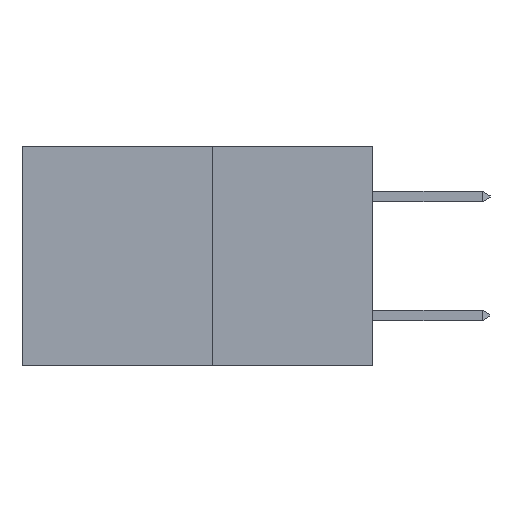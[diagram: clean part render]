
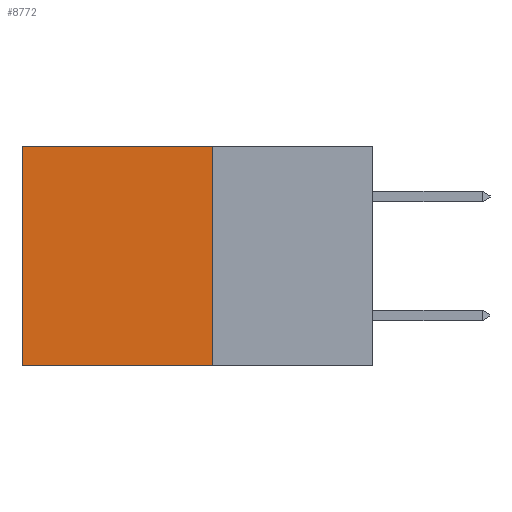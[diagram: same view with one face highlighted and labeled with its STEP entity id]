
A CAD part, left-side view. The second image highlights one B-rep face of the part: STEP entity #8772.
In plain terms, the highlighted planar face has unit normal (-1, 0, 0).
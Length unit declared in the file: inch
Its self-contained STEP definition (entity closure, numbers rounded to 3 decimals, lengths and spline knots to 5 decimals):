
#149 = VERTEX_POINT ( 'NONE', #5494 ) ;
#459 = ORIENTED_EDGE ( 'NONE', *, *, #4721, .F. ) ;
#1089 = VERTEX_POINT ( 'NONE', #6382 ) ;
#1174 = CARTESIAN_POINT ( 'NONE',  ( 0.277, 0.27, 0. ) ) ;
#1206 = CARTESIAN_POINT ( 'NONE',  ( 0.277, 0.27, -0.37 ) ) ;
#1286 = LINE ( 'NONE', #1206, #12986 ) ;
#1322 = EDGE_CURVE ( 'NONE', #11933, #1089, #7923, .T. ) ;
#1432 = CARTESIAN_POINT ( 'NONE',  ( 0.277, 0.59, 0. ) ) ;
#1662 = VECTOR ( 'NONE', #5779, 39.37008 ) ;
#2439 = CARTESIAN_POINT ( 'NONE',  ( 0.277, 0.27, -0.37 ) ) ;
#2505 = PLANE ( 'NONE',  #3910 ) ;
#2763 = EDGE_LOOP ( 'NONE', ( #3074, #7607, #459, #6108 ) ) ;
#2765 = VECTOR ( 'NONE', #7814, 39.37008 ) ;
#3074 = ORIENTED_EDGE ( 'NONE', *, *, #1322, .T. ) ;
#3130 = LINE ( 'NONE', #1174, #2765 ) ;
#3910 = AXIS2_PLACEMENT_3D ( 'NONE', #8044, #5910, #13481 ) ;
#4675 = VERTEX_POINT ( 'NONE', #2439 ) ;
#4721 = EDGE_CURVE ( 'NONE', #149, #4675, #7970, .T. ) ;
#5494 = CARTESIAN_POINT ( 'NONE',  ( 0.277, 0.27, 0. ) ) ;
#5779 = DIRECTION ( 'NONE',  ( 0., 0., -1. ) ) ;
#5814 = CARTESIAN_POINT ( 'NONE',  ( 0.277, 0.59, -0.37 ) ) ;
#5910 = DIRECTION ( 'NONE',  ( 1., 0., 0. ) ) ;
#6108 = ORIENTED_EDGE ( 'NONE', *, *, #8269, .T. ) ;
#6382 = CARTESIAN_POINT ( 'NONE',  ( 0.277, 0.59, -0.37 ) ) ;
#6928 = CARTESIAN_POINT ( 'NONE',  ( 0.277, 0.27, -0.37 ) ) ;
#7096 = DIRECTION ( 'NONE',  ( 0., 0., -1. ) ) ;
#7607 = ORIENTED_EDGE ( 'NONE', *, *, #8627, .F. ) ;
#7814 = DIRECTION ( 'NONE',  ( 0., 1., 0. ) ) ;
#7923 = LINE ( 'NONE', #5814, #1662 ) ;
#7970 = LINE ( 'NONE', #6928, #13721 ) ;
#8044 = CARTESIAN_POINT ( 'NONE',  ( 0.277, 0.27, -0.37 ) ) ;
#8269 = EDGE_CURVE ( 'NONE', #149, #11933, #3130, .T. ) ;
#8627 = EDGE_CURVE ( 'NONE', #4675, #1089, #1286, .T. ) ;
#8772 = ADVANCED_FACE ( 'NONE', ( #11258 ), #2505, .F. ) ;
#8973 = DIRECTION ( 'NONE',  ( 0., 1., 0. ) ) ;
#11258 = FACE_OUTER_BOUND ( 'NONE', #2763, .T. ) ;
#11933 = VERTEX_POINT ( 'NONE', #1432 ) ;
#12986 = VECTOR ( 'NONE', #8973, 39.37008 ) ;
#13481 = DIRECTION ( 'NONE',  ( 0., 0., -1. ) ) ;
#13721 = VECTOR ( 'NONE', #7096, 39.37008 ) ;
